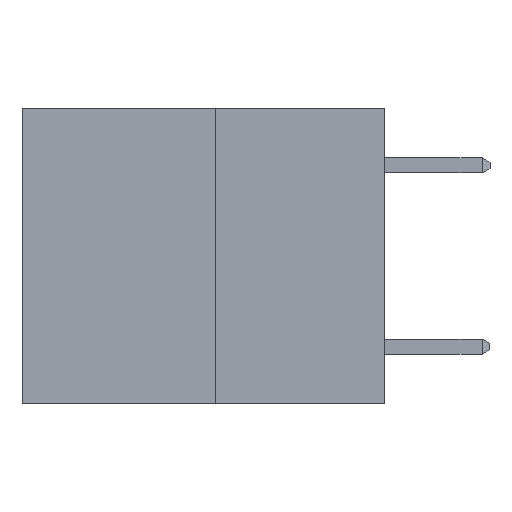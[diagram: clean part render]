
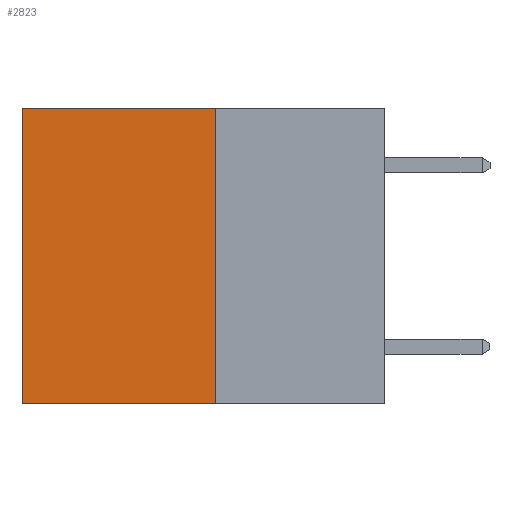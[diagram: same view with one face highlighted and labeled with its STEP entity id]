
A CAD part, left-side view. The second image highlights one B-rep face of the part: STEP entity #2823.
In plain terms, the highlighted planar face has unit normal (-1, 0, 0).
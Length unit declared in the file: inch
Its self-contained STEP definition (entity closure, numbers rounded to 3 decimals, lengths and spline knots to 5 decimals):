
#46 = CARTESIAN_POINT ( 'NONE',  ( 0.3165, 0.28, -0.49 ) ) ;
#1075 = VECTOR ( 'NONE', #8137, 39.37008 ) ;
#1307 = DIRECTION ( 'NONE',  ( 0., 0., -1. ) ) ;
#1428 = CARTESIAN_POINT ( 'NONE',  ( 0.3165, 0.6, -0.49 ) ) ;
#1620 = EDGE_CURVE ( 'NONE', #6275, #5261, #7209, .T. ) ;
#1804 = CARTESIAN_POINT ( 'NONE',  ( 0.3165, 0.28, -0.49 ) ) ;
#1877 = DIRECTION ( 'NONE',  ( 0., 0., -1. ) ) ;
#2297 = ORIENTED_EDGE ( 'NONE', *, *, #2382, .F. ) ;
#2382 = EDGE_CURVE ( 'NONE', #6275, #4555, #13259, .T. ) ;
#2823 = ADVANCED_FACE ( 'NONE', ( #7175 ), #10863, .F. ) ;
#3409 = EDGE_CURVE ( 'NONE', #5261, #5985, #6775, .T. ) ;
#4555 = VERTEX_POINT ( 'NONE', #8365 ) ;
#4728 = AXIS2_PLACEMENT_3D ( 'NONE', #46, #6168, #1307 ) ;
#5106 = DIRECTION ( 'NONE',  ( 0., 1., 0. ) ) ;
#5261 = VERTEX_POINT ( 'NONE', #7062 ) ;
#5413 = CARTESIAN_POINT ( 'NONE',  ( 0.3165, 0.28, 0. ) ) ;
#5985 = VERTEX_POINT ( 'NONE', #1428 ) ;
#6168 = DIRECTION ( 'NONE',  ( 1., 0., 0. ) ) ;
#6275 = VERTEX_POINT ( 'NONE', #5413 ) ;
#6775 = LINE ( 'NONE', #14321, #8655 ) ;
#6807 = LINE ( 'NONE', #1804, #1075 ) ;
#7062 = CARTESIAN_POINT ( 'NONE',  ( 0.3165, 0.6, 0. ) ) ;
#7175 = FACE_OUTER_BOUND ( 'NONE', #12837, .T. ) ;
#7209 = LINE ( 'NONE', #12121, #10035 ) ;
#8137 = DIRECTION ( 'NONE',  ( 0., 1., 0. ) ) ;
#8365 = CARTESIAN_POINT ( 'NONE',  ( 0.3165, 0.28, -0.49 ) ) ;
#8655 = VECTOR ( 'NONE', #12025, 39.37008 ) ;
#10035 = VECTOR ( 'NONE', #5106, 39.37008 ) ;
#10803 = ORIENTED_EDGE ( 'NONE', *, *, #14942, .F. ) ;
#10863 = PLANE ( 'NONE',  #4728 ) ;
#11607 = CARTESIAN_POINT ( 'NONE',  ( 0.3165, 0.28, -0.49 ) ) ;
#11639 = ORIENTED_EDGE ( 'NONE', *, *, #1620, .T. ) ;
#12025 = DIRECTION ( 'NONE',  ( 0., 0., -1. ) ) ;
#12121 = CARTESIAN_POINT ( 'NONE',  ( 0.3165, 0.28, 0. ) ) ;
#12594 = ORIENTED_EDGE ( 'NONE', *, *, #3409, .T. ) ;
#12837 = EDGE_LOOP ( 'NONE', ( #12594, #10803, #2297, #11639 ) ) ;
#13259 = LINE ( 'NONE', #11607, #14210 ) ;
#14210 = VECTOR ( 'NONE', #1877, 39.37008 ) ;
#14321 = CARTESIAN_POINT ( 'NONE',  ( 0.3165, 0.6, -0.49 ) ) ;
#14942 = EDGE_CURVE ( 'NONE', #4555, #5985, #6807, .T. ) ;
